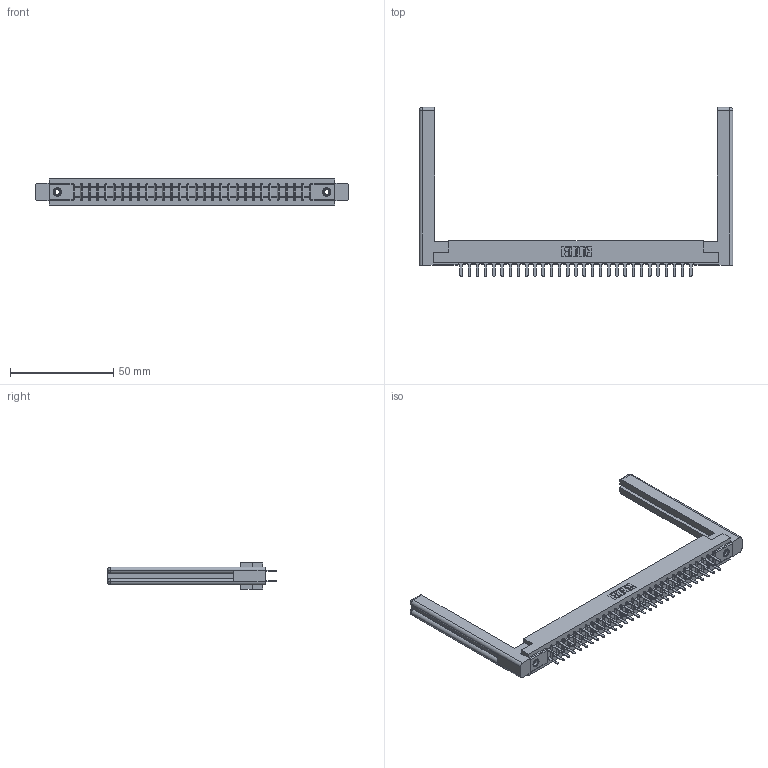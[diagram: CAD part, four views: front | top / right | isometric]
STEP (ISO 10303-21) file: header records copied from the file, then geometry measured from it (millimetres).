
FILE_DESCRIPTION (( 'STEP AP203' ), '1' );
FILE_NAME ('307-058-520-258.STEP', '2019-09-06T14:06:29', ( '' ), ( '' ), 'SwSTEP 2.0', 'SolidWorks 2016', '' );
FILE_SCHEMA (( 'CONFIG_CONTROL_DESIGN' ));
Length unit declared in the file: inch
Products named in the file (5): 307-058-520-258; 345-250-001_345-250-001-102; 307-220-058; 307-290-001_520; 307 Part_.156 Dia Mounting Holes
Assembly tree (63 placements, depth 2):
  307-058-520-258
    307 Part_.156 Dia Mounting Holes
    307-290-001_520  x58
    307-220-058  x2
    345-250-001_345-250-001-102  x2
Bounding box: 151.54 x 81.74 x 12.7 mm (x, y, z)
Volume: 23193.9 mm3; surface area: 24380.1 mm2
Topology: 63 solids, 63 shells, 2958 faces, 8217 edges, 5306 vertices
Faces by surface type: plane 1952, cylinder 922, sphere 60, torus 12, cone 12
Entity records: 29993 total; most frequent: CARTESIAN_POINT 4928, ORIENTED_EDGE 4824, DIRECTION 4790, EDGE_CURVE 2412, VECTOR 1842, LINE 1842, VERTEX_POINT 1558, AXIS2_PLACEMENT_3D 1474
